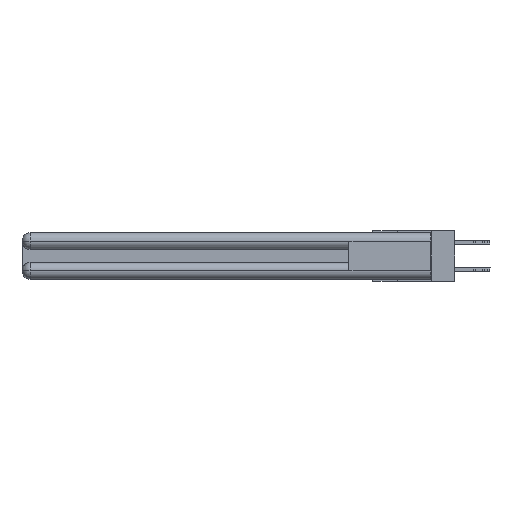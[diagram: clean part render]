
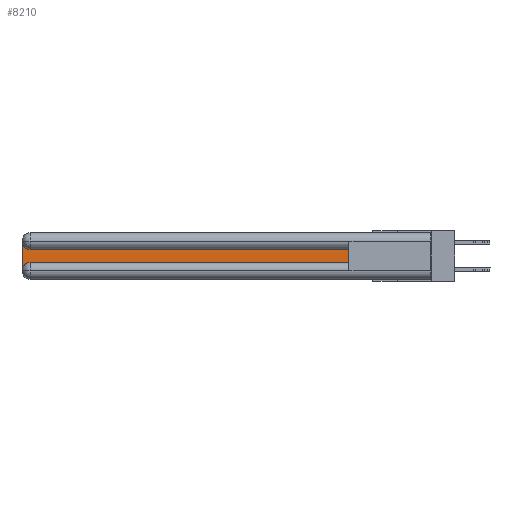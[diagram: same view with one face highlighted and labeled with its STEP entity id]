
A CAD part, left-side view. The second image highlights one B-rep face of the part: STEP entity #8210.
In plain terms, the highlighted planar face has unit normal (-1, 0, 0).
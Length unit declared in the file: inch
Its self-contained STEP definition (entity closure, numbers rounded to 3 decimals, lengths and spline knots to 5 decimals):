
#282 = ORIENTED_EDGE ( 'NONE', *, *, #6788, .T. ) ;
#584 = DIRECTION ( 'NONE',  ( 0., 0., 1. ) ) ;
#1461 = VERTEX_POINT ( 'NONE', #6184 ) ;
#1571 = CIRCLE ( 'NONE', #21903, 0.06 ) ;
#3045 = DIRECTION ( 'NONE',  ( 1., 0., 0. ) ) ;
#3709 = CARTESIAN_POINT ( 'NONE',  ( 0.075, 2.94, -0.0625 ) ) ;
#5023 = CARTESIAN_POINT ( 'NONE',  ( 0.075, 0.6, -0.2175 ) ) ;
#5458 = CARTESIAN_POINT ( 'NONE',  ( 0.075, 2.94, -0.1225 ) ) ;
#5786 = DIRECTION ( 'NONE',  ( 0., -1., 0. ) ) ;
#6184 = CARTESIAN_POINT ( 'NONE',  ( 0.075, 0.6, -0.1225 ) ) ;
#6788 = EDGE_CURVE ( 'NONE', #11453, #1461, #9979, .T. ) ;
#7329 = CARTESIAN_POINT ( 'NONE',  ( 0.075, 0.6, -0.1225 ) ) ;
#7356 = CARTESIAN_POINT ( 'NONE',  ( 0.075, 2.94, -0.2175 ) ) ;
#7409 = AXIS2_PLACEMENT_3D ( 'NONE', #8260, #17096, #19314 ) ;
#7448 = AXIS2_PLACEMENT_3D ( 'NONE', #16358, #3045, #20768 ) ;
#7728 = VERTEX_POINT ( 'NONE', #5458 ) ;
#7926 = DIRECTION ( 'NONE',  ( 1., 0., 0. ) ) ;
#8210 = ADVANCED_FACE ( 'NONE', ( #24014 ), #11887, .F. ) ;
#8224 = VECTOR ( 'NONE', #17995, 39.37008 ) ;
#8260 = CARTESIAN_POINT ( 'NONE',  ( 0.075, 2.94, -0.2775 ) ) ;
#8990 = CARTESIAN_POINT ( 'NONE',  ( 0.075, 3., -0.2175 ) ) ;
#9305 = EDGE_CURVE ( 'NONE', #9711, #11453, #16448, .T. ) ;
#9711 = VERTEX_POINT ( 'NONE', #7356 ) ;
#9942 = LINE ( 'NONE', #8990, #8224 ) ;
#9979 = LINE ( 'NONE', #20584, #14495 ) ;
#10061 = ORIENTED_EDGE ( 'NONE', *, *, #25297, .T. ) ;
#10103 = LINE ( 'NONE', #7329, #20846 ) ;
#11296 = ORIENTED_EDGE ( 'NONE', *, *, #9305, .T. ) ;
#11453 = VERTEX_POINT ( 'NONE', #5023 ) ;
#11887 = PLANE ( 'NONE',  #7448 ) ;
#14495 = VECTOR ( 'NONE', #584, 39.37008 ) ;
#14846 = CARTESIAN_POINT ( 'NONE',  ( 0.075, 3., -0.0625 ) ) ;
#15937 = EDGE_CURVE ( 'NONE', #1461, #7728, #10103, .T. ) ;
#16132 = ORIENTED_EDGE ( 'NONE', *, *, #18979, .T. ) ;
#16358 = CARTESIAN_POINT ( 'NONE',  ( 0.075, 3., -0.1225 ) ) ;
#16448 = LINE ( 'NONE', #27619, #19206 ) ;
#17096 = DIRECTION ( 'NONE',  ( 1., 0., 0. ) ) ;
#17750 = VERTEX_POINT ( 'NONE', #24256 ) ;
#17879 = CIRCLE ( 'NONE', #7409, 0.06 ) ;
#17975 = EDGE_CURVE ( 'NONE', #24240, #17750, #9942, .T. ) ;
#17995 = DIRECTION ( 'NONE',  ( 0., 0., -1. ) ) ;
#18979 = EDGE_CURVE ( 'NONE', #17750, #9711, #17879, .T. ) ;
#19124 = EDGE_LOOP ( 'NONE', ( #24949, #10061, #23029, #16132, #11296, #282 ) ) ;
#19206 = VECTOR ( 'NONE', #5786, 39.37008 ) ;
#19239 = DIRECTION ( 'NONE',  ( 0., 0., -1. ) ) ;
#19314 = DIRECTION ( 'NONE',  ( 0., 0., -1. ) ) ;
#20584 = CARTESIAN_POINT ( 'NONE',  ( 0.075, 0.6, -0.2175 ) ) ;
#20768 = DIRECTION ( 'NONE',  ( 0., 0., -1. ) ) ;
#20846 = VECTOR ( 'NONE', #22501, 39.37008 ) ;
#21903 = AXIS2_PLACEMENT_3D ( 'NONE', #3709, #7926, #19239 ) ;
#22501 = DIRECTION ( 'NONE',  ( 0., 1., 0. ) ) ;
#23029 = ORIENTED_EDGE ( 'NONE', *, *, #17975, .T. ) ;
#24014 = FACE_OUTER_BOUND ( 'NONE', #19124, .T. ) ;
#24240 = VERTEX_POINT ( 'NONE', #14846 ) ;
#24256 = CARTESIAN_POINT ( 'NONE',  ( 0.075, 3., -0.2775 ) ) ;
#24949 = ORIENTED_EDGE ( 'NONE', *, *, #15937, .T. ) ;
#25297 = EDGE_CURVE ( 'NONE', #7728, #24240, #1571, .T. ) ;
#27619 = CARTESIAN_POINT ( 'NONE',  ( 0.075, 0.6, -0.2175 ) ) ;
